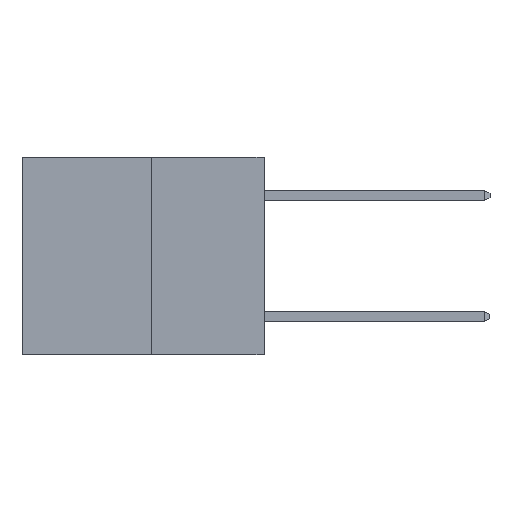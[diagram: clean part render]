
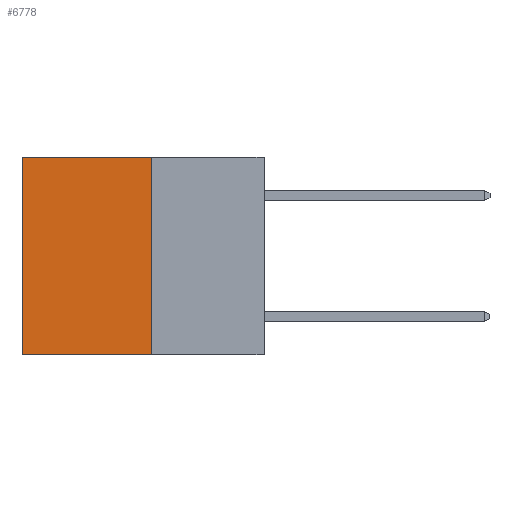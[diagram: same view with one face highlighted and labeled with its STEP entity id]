
A CAD part, left-side view. The second image highlights one B-rep face of the part: STEP entity #6778.
In plain terms, the highlighted planar face has unit normal (-1, 0, 0).
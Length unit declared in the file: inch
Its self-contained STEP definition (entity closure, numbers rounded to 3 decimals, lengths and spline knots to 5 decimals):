
#90 = VERTEX_POINT ( 'NONE', #6040 ) ;
#165 = DIRECTION ( 'NONE',  ( 0., 1., 0. ) ) ;
#1754 = EDGE_CURVE ( 'NONE', #90, #5913, #6220, .T. ) ;
#2017 = DIRECTION ( 'NONE',  ( 1., 0., 0. ) ) ;
#2952 = EDGE_CURVE ( 'NONE', #7252, #10907, #2985, .T. ) ;
#2985 = LINE ( 'NONE', #11521, #10807 ) ;
#4404 = CARTESIAN_POINT ( 'NONE',  ( 0.3165, 0.28, 0. ) ) ;
#5051 = AXIS2_PLACEMENT_3D ( 'NONE', #7960, #2017, #8073 ) ;
#5594 = ORIENTED_EDGE ( 'NONE', *, *, #14212, .T. ) ;
#5684 = CARTESIAN_POINT ( 'NONE',  ( 0.3165, 0.6, -0.49 ) ) ;
#5780 = ORIENTED_EDGE ( 'NONE', *, *, #2952, .F. ) ;
#5913 = VERTEX_POINT ( 'NONE', #12435 ) ;
#6040 = CARTESIAN_POINT ( 'NONE',  ( 0.3165, 0.28, 0. ) ) ;
#6220 = LINE ( 'NONE', #4404, #14604 ) ;
#6778 = ADVANCED_FACE ( 'NONE', ( #11833 ), #9372, .F. ) ;
#7252 = VERTEX_POINT ( 'NONE', #11652 ) ;
#7819 = LINE ( 'NONE', #9407, #9929 ) ;
#7891 = DIRECTION ( 'NONE',  ( 0., 1., 0. ) ) ;
#7960 = CARTESIAN_POINT ( 'NONE',  ( 0.3165, 0.28, -0.49 ) ) ;
#7994 = DIRECTION ( 'NONE',  ( 0., 0., -1. ) ) ;
#8073 = DIRECTION ( 'NONE',  ( 0., 0., -1. ) ) ;
#9333 = CARTESIAN_POINT ( 'NONE',  ( 0.3165, 0.28, -0.49 ) ) ;
#9372 = PLANE ( 'NONE',  #5051 ) ;
#9407 = CARTESIAN_POINT ( 'NONE',  ( 0.3165, 0.6, -0.49 ) ) ;
#9929 = VECTOR ( 'NONE', #7994, 39.37008 ) ;
#9957 = LINE ( 'NONE', #9333, #12431 ) ;
#10807 = VECTOR ( 'NONE', #165, 39.37008 ) ;
#10907 = VERTEX_POINT ( 'NONE', #5684 ) ;
#11521 = CARTESIAN_POINT ( 'NONE',  ( 0.3165, 0.28, -0.49 ) ) ;
#11652 = CARTESIAN_POINT ( 'NONE',  ( 0.3165, 0.28, -0.49 ) ) ;
#11833 = FACE_OUTER_BOUND ( 'NONE', #12725, .T. ) ;
#12431 = VECTOR ( 'NONE', #13600, 39.37008 ) ;
#12435 = CARTESIAN_POINT ( 'NONE',  ( 0.3165, 0.6, 0. ) ) ;
#12725 = EDGE_LOOP ( 'NONE', ( #5594, #5780, #12833, #14506 ) ) ;
#12833 = ORIENTED_EDGE ( 'NONE', *, *, #13686, .F. ) ;
#13600 = DIRECTION ( 'NONE',  ( 0., 0., -1. ) ) ;
#13686 = EDGE_CURVE ( 'NONE', #90, #7252, #9957, .T. ) ;
#14212 = EDGE_CURVE ( 'NONE', #5913, #10907, #7819, .T. ) ;
#14506 = ORIENTED_EDGE ( 'NONE', *, *, #1754, .T. ) ;
#14604 = VECTOR ( 'NONE', #7891, 39.37008 ) ;
